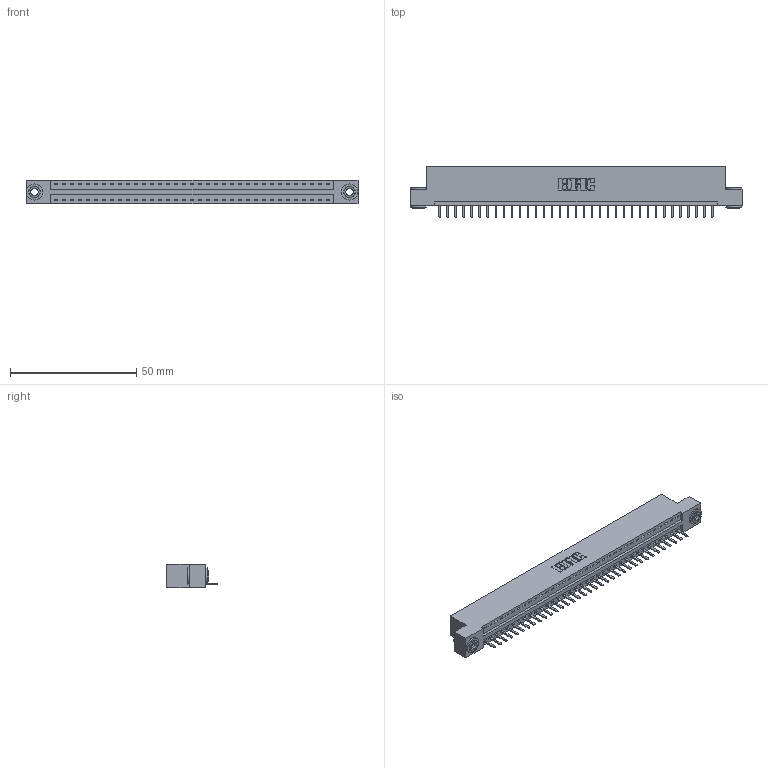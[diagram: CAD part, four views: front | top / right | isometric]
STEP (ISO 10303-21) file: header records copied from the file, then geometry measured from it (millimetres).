
FILE_DESCRIPTION (( 'STEP AP203' ), '1' );
FILE_NAME ('396-035-520-103.STEP', '2018-09-06T02:07:10', ( '' ), ( '' ), 'SwSTEP 2.0', 'SolidWorks 2016', '' );
FILE_SCHEMA (( 'CONFIG_CONTROL_DESIGN' ));
Length unit declared in the file: inch
Products named in the file (4): 346 Part_Flush Mounting Lugs - 0.156 Dia-TH; 345-292-001_345-293-120; 345-250-002_345-250-002-102; 396-035-520-103
Assembly tree (38 placements, depth 2):
  396-035-520-103
    346 Part_Flush Mounting Lugs - 0.156 Dia-TH
    345-292-001_345-293-120  x35
    345-250-002_345-250-002-102  x2
Bounding box: 131.7 x 20.02 x 9.4 mm (x, y, z)
Volume: 12477 mm3; surface area: 15402.2 mm2
Topology: 38 solids, 38 shells, 2330 faces, 6845 edges, 4466 vertices
Faces by surface type: plane 1556, cylinder 766, cone 8
Entity records: 23428 total; most frequent: CARTESIAN_POINT 4008, ORIENTED_EDGE 3958, DIRECTION 3563, EDGE_CURVE 1979, VECTOR 1679, LINE 1679, VERTEX_POINT 1314, AXIS2_PLACEMENT_3D 942
